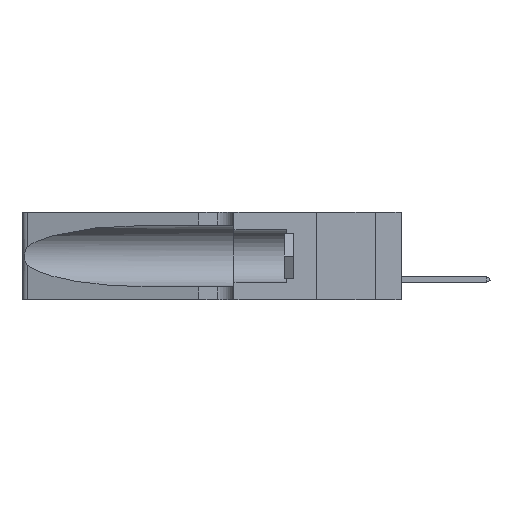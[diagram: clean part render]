
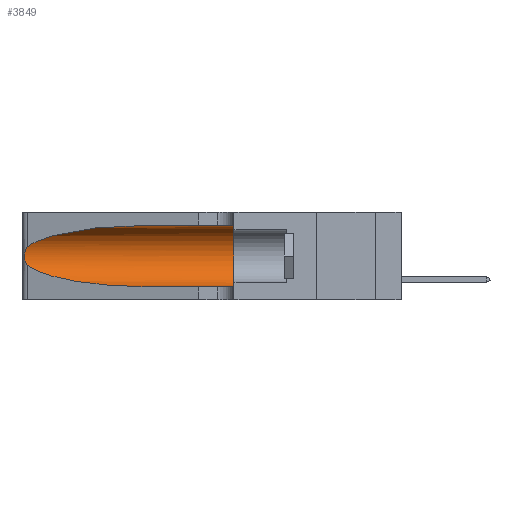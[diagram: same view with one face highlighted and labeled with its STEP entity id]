
A CAD part, left-side view. The second image highlights one B-rep face of the part: STEP entity #3849.
In plain terms, the highlighted cylindrical face has radius 3.308 mm (diameter 6.617 mm), a partial arc.
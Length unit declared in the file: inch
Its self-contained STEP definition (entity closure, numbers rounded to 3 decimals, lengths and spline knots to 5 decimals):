
#94 = DIRECTION ( 'NONE',  ( 0., -1., 0. ) ) ;
#1113 = CARTESIAN_POINT ( 'NONE',  ( 0.25555, 1.22993, 0.14849 ) ) ;
#1930 = CARTESIAN_POINT ( 'NONE',  ( 0.1305, 1.61858, 0.31525 ) ) ;
#2362 = ORIENTED_EDGE ( 'NONE', *, *, #7938, .T. ) ;
#2447 = CARTESIAN_POINT ( 'NONE',  ( 0.1305, 1.61858, 0.185 ) ) ;
#2458 = VERTEX_POINT ( 'NONE', #19520 ) ;
#3144 = CARTESIAN_POINT ( 'NONE',  ( 0.26017, 1.23833, 0.17102 ) ) ;
#3249 = CARTESIAN_POINT ( 'NONE',  ( 0.25639, 1.23186, 0.15144 ) ) ;
#3849 = ADVANCED_FACE ( 'NONE', ( #25193 ), #26285, .F. ) ;
#4189 = CARTESIAN_POINT ( 'NONE',  ( 0.1305, 0.72297, 0.05475 ) ) ;
#4246 = VERTEX_POINT ( 'NONE', #5523 ) ;
#4390 = ORIENTED_EDGE ( 'NONE', *, *, #11488, .F. ) ;
#4481 = CARTESIAN_POINT ( 'NONE',  ( 0.25487, 1.22718, 0.22369 ) ) ;
#5154 = CARTESIAN_POINT ( 'NONE',  ( 0.25487, 1.22718, 0.14631 ) ) ;
#5493 = CARTESIAN_POINT ( 'NONE',  ( 0.25856, 1.23593, 0.16098 ) ) ;
#5523 = CARTESIAN_POINT ( 'NONE',  ( 0.1305, 0.35, 0.31525 ) ) ;
#5812 = VECTOR ( 'NONE', #9301, 39.37008 ) ;
#6096 = CARTESIAN_POINT ( 'NONE',  ( 0.25487, 1.22718, 0.14631 ) ) ;
#6182 = VERTEX_POINT ( 'NONE', #13352 ) ;
#6391 = ORIENTED_EDGE ( 'NONE', *, *, #29060, .F. ) ;
#7065 = VERTEX_POINT ( 'NONE', #22874 ) ;
#7917 = CARTESIAN_POINT ( 'NONE',  ( 0.26018, 1.23835, 0.19895 ) ) ;
#7938 = EDGE_CURVE ( 'NONE', #25701, #24230, #12049, .T. ) ;
#8281 = AXIS2_PLACEMENT_3D ( 'NONE', #2447, #94, #23550 ) ;
#9031 = AXIS2_PLACEMENT_3D ( 'NONE', #29972, #15763, #22776 ) ;
#9114 = CARTESIAN_POINT ( 'NONE',  ( 0.18966, 0.96281, 0.31525 ) ) ;
#9301 = DIRECTION ( 'NONE',  ( 0., -1., 0. ) ) ;
#9419 = ORIENTED_EDGE ( 'NONE', *, *, #27553, .T. ) ;
#10170 = CARTESIAN_POINT ( 'NONE',  ( 0.25639, 1.23184, 0.21858 ) ) ;
#11276 = CARTESIAN_POINT ( 'NONE',  ( 0.2373, 1.15595, 0.28018 ) ) ;
#11488 = EDGE_CURVE ( 'NONE', #2458, #4246, #29233, .T. ) ;
#12049 =( BOUNDED_CURVE ( )  B_SPLINE_CURVE ( 3, ( #13044, #29556, #15553, #4189 ),
 .UNSPECIFIED., .F., .F. ) 
 B_SPLINE_CURVE_WITH_KNOTS ( ( 4, 4 ),
 ( 3.44316, 4.71239 ),
 .UNSPECIFIED. ) 
 CURVE ( )  GEOMETRIC_REPRESENTATION_ITEM ( )  RATIONAL_B_SPLINE_CURVE ( ( 1., 0.87, 0.87, 1. ) ) 
 REPRESENTATION_ITEM ( '' )  );
#12124 = CARTESIAN_POINT ( 'NONE',  ( 0.26075, 1.23896, 0.178 ) ) ;
#12228 = CARTESIAN_POINT ( 'NONE',  ( 0.25787, 1.23484, 0.2124 ) ) ;
#12524 = CARTESIAN_POINT ( 'NONE',  ( 0.25789, 1.23486, 0.15765 ) ) ;
#12941 = EDGE_CURVE ( 'NONE', #24230, #6182, #24403, .T. ) ;
#13044 = CARTESIAN_POINT ( 'NONE',  ( 0.25487, 1.22718, 0.14631 ) ) ;
#13352 = CARTESIAN_POINT ( 'NONE',  ( 0.1305, 0.35, 0.05475 ) ) ;
#14310 = VECTOR ( 'NONE', #16058, 39.37008 ) ;
#14386 = ORIENTED_EDGE ( 'NONE', *, *, #12941, .T. ) ;
#14803 = CARTESIAN_POINT ( 'NONE',  ( 0.26075, 1.23896, 0.19203 ) ) ;
#15553 = CARTESIAN_POINT ( 'NONE',  ( 0.18966, 0.96281, 0.05475 ) ) ;
#15763 = DIRECTION ( 'NONE',  ( 0., 1., 0. ) ) ;
#16058 = DIRECTION ( 'NONE',  ( 0., -1., 0. ) ) ;
#17144 = B_SPLINE_CURVE_WITH_KNOTS ( 'NONE', 3,
 ( #21738, #24141, #10170, #12228, #26495, #7917, #14803, #12124, #3144, #5493, #12524, #3249, #1113, #6096 ),
 .UNSPECIFIED., .F., .F.,
 ( 4, 2, 2, 2, 2, 2, 4 ),
 ( 0., 0.00027, 0.00053, 0.00107, 0.0016, 0.00187, 0.00214 ),
 .UNSPECIFIED. ) ;
#17651 = CARTESIAN_POINT ( 'NONE',  ( 0.1305, 0.72297, 0.31525 ) ) ;
#17897 = EDGE_LOOP ( 'NONE', ( #23175, #9419, #2362, #14386, #6391, #4390 ) ) ;
#19520 = CARTESIAN_POINT ( 'NONE',  ( 0.1305, 0.72297, 0.31525 ) ) ;
#21738 = CARTESIAN_POINT ( 'NONE',  ( 0.25487, 1.22718, 0.22369 ) ) ;
#21996 =( BOUNDED_CURVE ( )  B_SPLINE_CURVE ( 3, ( #17651, #9114, #11276, #4481 ),
 .UNSPECIFIED., .F., .F. ) 
 B_SPLINE_CURVE_WITH_KNOTS ( ( 4, 4 ),
 ( 1.5708, 2.84003 ),
 .UNSPECIFIED. ) 
 CURVE ( )  GEOMETRIC_REPRESENTATION_ITEM ( )  RATIONAL_B_SPLINE_CURVE ( ( 1., 0.87, 0.87, 1. ) ) 
 REPRESENTATION_ITEM ( '' )  );
#22776 = DIRECTION ( 'NONE',  ( 0., 0., 1. ) ) ;
#22874 = CARTESIAN_POINT ( 'NONE',  ( 0.25487, 1.22718, 0.22369 ) ) ;
#23175 = ORIENTED_EDGE ( 'NONE', *, *, #27024, .T. ) ;
#23386 = CARTESIAN_POINT ( 'NONE',  ( 0.1305, 1.61858, 0.05475 ) ) ;
#23550 = DIRECTION ( 'NONE',  ( 0., 0., -1. ) ) ;
#24141 = CARTESIAN_POINT ( 'NONE',  ( 0.25555, 1.22994, 0.2215 ) ) ;
#24230 = VERTEX_POINT ( 'NONE', #25906 ) ;
#24403 = LINE ( 'NONE', #23386, #5812 ) ;
#25193 = FACE_OUTER_BOUND ( 'NONE', #17897, .T. ) ;
#25701 = VERTEX_POINT ( 'NONE', #5154 ) ;
#25906 = CARTESIAN_POINT ( 'NONE',  ( 0.1305, 0.72297, 0.05475 ) ) ;
#26285 = CYLINDRICAL_SURFACE ( 'NONE', #8281, 0.13025 ) ;
#26495 = CARTESIAN_POINT ( 'NONE',  ( 0.25854, 1.2359, 0.20912 ) ) ;
#27024 = EDGE_CURVE ( 'NONE', #2458, #7065, #21996, .T. ) ;
#27553 = EDGE_CURVE ( 'NONE', #7065, #25701, #17144, .T. ) ;
#27968 = CIRCLE ( 'NONE', #9031, 0.13025 ) ;
#29060 = EDGE_CURVE ( 'NONE', #4246, #6182, #27968, .T. ) ;
#29233 = LINE ( 'NONE', #1930, #14310 ) ;
#29556 = CARTESIAN_POINT ( 'NONE',  ( 0.2373, 1.15595, 0.08982 ) ) ;
#29972 = CARTESIAN_POINT ( 'NONE',  ( 0.1305, 0.35, 0.185 ) ) ;
